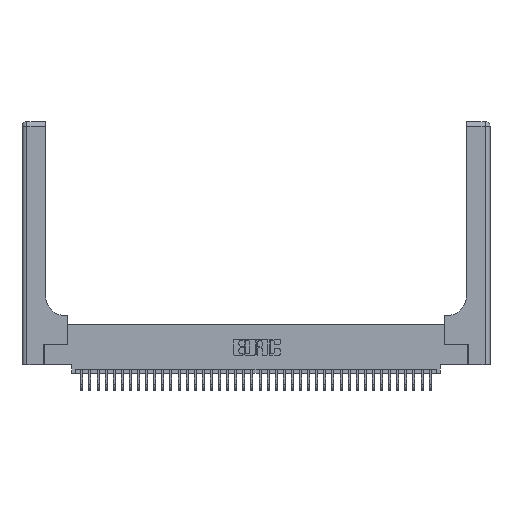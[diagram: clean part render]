
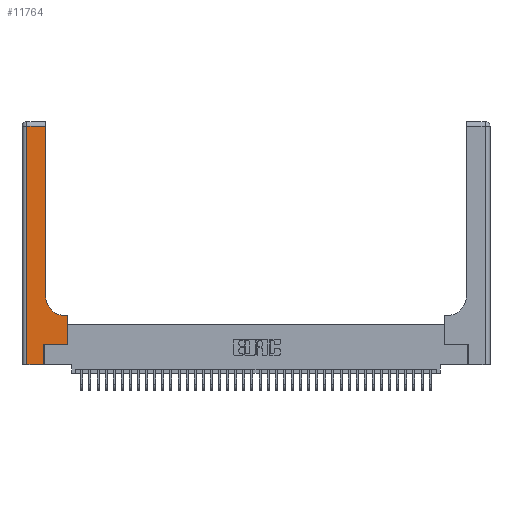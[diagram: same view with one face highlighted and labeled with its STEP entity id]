
A CAD part, top view. The second image highlights one B-rep face of the part: STEP entity #11764.
In plain terms, the highlighted planar face has unit normal (0, 0, 1).
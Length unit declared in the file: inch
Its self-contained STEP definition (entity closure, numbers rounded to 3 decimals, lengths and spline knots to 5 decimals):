
#136 = CARTESIAN_POINT ( 'NONE',  ( 0.2915, 2.94, 0.37 ) ) ;
#180 = VECTOR ( 'NONE', #28220, 39.37008 ) ;
#442 = DIRECTION ( 'NONE',  ( 1., 0., 0. ) ) ;
#955 = VERTEX_POINT ( 'NONE', #17821 ) ;
#1134 = VECTOR ( 'NONE', #31406, 39.37008 ) ;
#1911 = CARTESIAN_POINT ( 'NONE',  ( 0.5585, 0.25, 0.37 ) ) ;
#2395 = VECTOR ( 'NONE', #26505, 39.37008 ) ;
#2877 = CARTESIAN_POINT ( 'NONE',  ( 0.2915, 3., 0.37 ) ) ;
#3464 = LINE ( 'NONE', #7747, #12941 ) ;
#5511 = DIRECTION ( 'NONE',  ( -1., 0., 0. ) ) ;
#5555 = EDGE_CURVE ( 'NONE', #955, #39013, #8429, .T. ) ;
#5591 = AXIS2_PLACEMENT_3D ( 'NONE', #16450, #6742, #442 ) ;
#6158 = ORIENTED_EDGE ( 'NONE', *, *, #26005, .T. ) ;
#6720 = AXIS2_PLACEMENT_3D ( 'NONE', #33531, #17810, #37865 ) ;
#6742 = DIRECTION ( 'NONE',  ( 0., 0., -1. ) ) ;
#7188 = CARTESIAN_POINT ( 'NONE',  ( 0., 2.94, 0.37 ) ) ;
#7747 = CARTESIAN_POINT ( 'NONE',  ( 0.2915, 0.6, 0.37 ) ) ;
#8429 = LINE ( 'NONE', #25238, #26813 ) ;
#10876 = LINE ( 'NONE', #7188, #2395 ) ;
#11360 = DIRECTION ( 'NONE',  ( 1., 0., 0. ) ) ;
#11764 = ADVANCED_FACE ( 'NONE', ( #26890 ), #33971, .F. ) ;
#12109 = LINE ( 'NONE', #21977, #180 ) ;
#12674 = VERTEX_POINT ( 'NONE', #34322 ) ;
#12941 = VECTOR ( 'NONE', #5511, 39.37008 ) ;
#13299 = CARTESIAN_POINT ( 'NONE',  ( 0.5585, 0.6, 0.37 ) ) ;
#13917 = CARTESIAN_POINT ( 'NONE',  ( 0.2915, 0.85, 0.37 ) ) ;
#16450 = CARTESIAN_POINT ( 'NONE',  ( 0.5415, 0.85, 0.37 ) ) ;
#16764 = EDGE_CURVE ( 'NONE', #28016, #955, #12109, .T. ) ;
#17810 = DIRECTION ( 'NONE',  ( 0., 0., -1. ) ) ;
#17815 = VERTEX_POINT ( 'NONE', #24903 ) ;
#17821 = CARTESIAN_POINT ( 'NONE',  ( 0.269, 0.25, 0.37 ) ) ;
#18252 = LINE ( 'NONE', #30414, #35675 ) ;
#18358 = EDGE_LOOP ( 'NONE', ( #24133, #6158, #23226, #24900, #28698, #29377, #31421, #31404, #25216 ) ) ;
#18537 = LINE ( 'NONE', #2877, #1134 ) ;
#19055 = VECTOR ( 'NONE', #24308, 39.37008 ) ;
#19324 = CIRCLE ( 'NONE', #5591, 0.25 ) ;
#20827 = EDGE_CURVE ( 'NONE', #39013, #35552, #27475, .T. ) ;
#20831 = DIRECTION ( 'NONE',  ( 0., -1., 0. ) ) ;
#21977 = CARTESIAN_POINT ( 'NONE',  ( 0.269, 0., 0.37 ) ) ;
#22030 = EDGE_CURVE ( 'NONE', #35552, #12674, #3464, .T. ) ;
#23226 = ORIENTED_EDGE ( 'NONE', *, *, #35093, .T. ) ;
#24133 = ORIENTED_EDGE ( 'NONE', *, *, #40576, .T. ) ;
#24308 = DIRECTION ( 'NONE',  ( 0., 1., 0. ) ) ;
#24900 = ORIENTED_EDGE ( 'NONE', *, *, #30394, .T. ) ;
#24903 = CARTESIAN_POINT ( 'NONE',  ( 0.06, 2.94, 0.37 ) ) ;
#25216 = ORIENTED_EDGE ( 'NONE', *, *, #26588, .T. ) ;
#25238 = CARTESIAN_POINT ( 'NONE',  ( 0.269, 0.25, 0.37 ) ) ;
#25918 = LINE ( 'NONE', #27201, #30380 ) ;
#26005 = EDGE_CURVE ( 'NONE', #34709, #17815, #10876, .T. ) ;
#26505 = DIRECTION ( 'NONE',  ( -1., 0., 0. ) ) ;
#26588 = EDGE_CURVE ( 'NONE', #12674, #38977, #19324, .T. ) ;
#26813 = VECTOR ( 'NONE', #35832, 39.37008 ) ;
#26890 = FACE_OUTER_BOUND ( 'NONE', #18358, .T. ) ;
#27201 = CARTESIAN_POINT ( 'NONE',  ( 0., 0., 0.37 ) ) ;
#27475 = LINE ( 'NONE', #1911, #19055 ) ;
#28016 = VERTEX_POINT ( 'NONE', #36694 ) ;
#28220 = DIRECTION ( 'NONE',  ( 0., 1., 0. ) ) ;
#28478 = CARTESIAN_POINT ( 'NONE',  ( 0.06, 0., 0.37 ) ) ;
#28698 = ORIENTED_EDGE ( 'NONE', *, *, #16764, .T. ) ;
#29377 = ORIENTED_EDGE ( 'NONE', *, *, #5555, .T. ) ;
#30380 = VECTOR ( 'NONE', #11360, 39.37008 ) ;
#30394 = EDGE_CURVE ( 'NONE', #35381, #28016, #25918, .T. ) ;
#30414 = CARTESIAN_POINT ( 'NONE',  ( 0.06, 3., 0.37 ) ) ;
#31404 = ORIENTED_EDGE ( 'NONE', *, *, #22030, .T. ) ;
#31406 = DIRECTION ( 'NONE',  ( 0., 1., 0. ) ) ;
#31421 = ORIENTED_EDGE ( 'NONE', *, *, #20827, .T. ) ;
#33531 = CARTESIAN_POINT ( 'NONE',  ( 0., 3., 0.37 ) ) ;
#33971 = PLANE ( 'NONE',  #6720 ) ;
#34322 = CARTESIAN_POINT ( 'NONE',  ( 0.5415, 0.6, 0.37 ) ) ;
#34709 = VERTEX_POINT ( 'NONE', #136 ) ;
#35093 = EDGE_CURVE ( 'NONE', #17815, #35381, #18252, .T. ) ;
#35381 = VERTEX_POINT ( 'NONE', #28478 ) ;
#35552 = VERTEX_POINT ( 'NONE', #13299 ) ;
#35675 = VECTOR ( 'NONE', #20831, 39.37008 ) ;
#35832 = DIRECTION ( 'NONE',  ( 1., 0., 0. ) ) ;
#36442 = CARTESIAN_POINT ( 'NONE',  ( 0.5585, 0.25, 0.37 ) ) ;
#36694 = CARTESIAN_POINT ( 'NONE',  ( 0.269, 0., 0.37 ) ) ;
#37865 = DIRECTION ( 'NONE',  ( -1., 0., 0. ) ) ;
#38977 = VERTEX_POINT ( 'NONE', #13917 ) ;
#39013 = VERTEX_POINT ( 'NONE', #36442 ) ;
#40576 = EDGE_CURVE ( 'NONE', #38977, #34709, #18537, .T. ) ;
